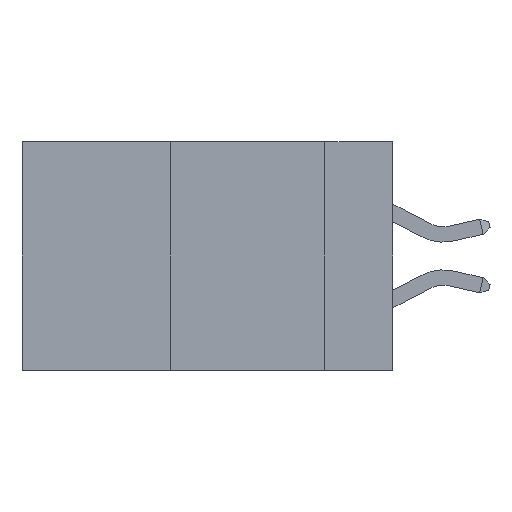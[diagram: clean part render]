
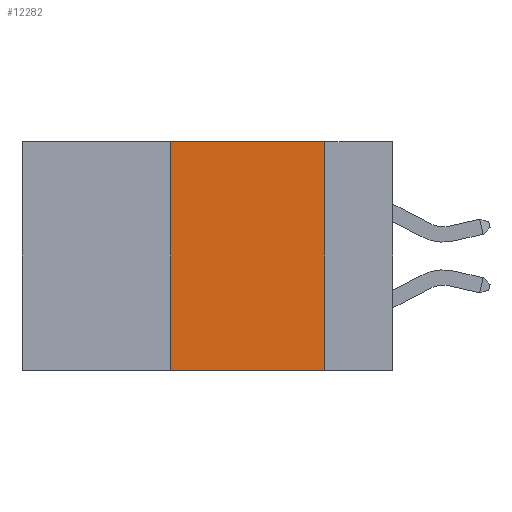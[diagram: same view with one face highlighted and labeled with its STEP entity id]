
A CAD part, left-side view. The second image highlights one B-rep face of the part: STEP entity #12282.
In plain terms, the highlighted planar face has unit normal (-1, 0, 0).
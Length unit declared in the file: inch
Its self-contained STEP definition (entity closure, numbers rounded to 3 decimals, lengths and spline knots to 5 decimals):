
#182 = LINE ( 'NONE', #2516, #6901 ) ;
#681 = CARTESIAN_POINT ( 'NONE',  ( 0., 0.6, -0.37 ) ) ;
#2028 = ORIENTED_EDGE ( 'NONE', *, *, #19809, .F. ) ;
#2516 = CARTESIAN_POINT ( 'NONE',  ( 0., 0.6, 0. ) ) ;
#3698 = VERTEX_POINT ( 'NONE', #8762 ) ;
#4005 = VERTEX_POINT ( 'NONE', #12855 ) ;
#5196 = ORIENTED_EDGE ( 'NONE', *, *, #9722, .F. ) ;
#5280 = ORIENTED_EDGE ( 'NONE', *, *, #16238, .F. ) ;
#5758 = ORIENTED_EDGE ( 'NONE', *, *, #14115, .T. ) ;
#6901 = VECTOR ( 'NONE', #9840, 39.37008 ) ;
#7137 = VERTEX_POINT ( 'NONE', #12231 ) ;
#8507 = PLANE ( 'NONE',  #9341 ) ;
#8762 = CARTESIAN_POINT ( 'NONE',  ( 0., 0.11, -0.37 ) ) ;
#8833 = VECTOR ( 'NONE', #22414, 39.37008 ) ;
#9341 = AXIS2_PLACEMENT_3D ( 'NONE', #16001, #14128, #17877 ) ;
#9382 = LINE ( 'NONE', #16503, #16396 ) ;
#9722 = EDGE_CURVE ( 'NONE', #7137, #4005, #14652, .T. ) ;
#9840 = DIRECTION ( 'NONE',  ( 0., -1., 0. ) ) ;
#11638 = FACE_OUTER_BOUND ( 'NONE', #14631, .T. ) ;
#12231 = CARTESIAN_POINT ( 'NONE',  ( 0., 0.36, -0.37 ) ) ;
#12282 = ADVANCED_FACE ( 'NONE', ( #11638 ), #8507, .F. ) ;
#12676 = DIRECTION ( 'NONE',  ( 0., 0., -1. ) ) ;
#12855 = CARTESIAN_POINT ( 'NONE',  ( 0., 0.36, 0. ) ) ;
#13872 = DIRECTION ( 'NONE',  ( 0., -1., 0. ) ) ;
#14115 = EDGE_CURVE ( 'NONE', #7137, #3698, #17105, .T. ) ;
#14128 = DIRECTION ( 'NONE',  ( 1., 0., 0. ) ) ;
#14631 = EDGE_LOOP ( 'NONE', ( #5280, #2028, #5196, #5758 ) ) ;
#14652 = LINE ( 'NONE', #20379, #8833 ) ;
#15928 = VERTEX_POINT ( 'NONE', #15932 ) ;
#15932 = CARTESIAN_POINT ( 'NONE',  ( 0., 0.11, 0. ) ) ;
#16001 = CARTESIAN_POINT ( 'NONE',  ( 0., 0.6, 0. ) ) ;
#16238 = EDGE_CURVE ( 'NONE', #15928, #3698, #9382, .T. ) ;
#16396 = VECTOR ( 'NONE', #12676, 39.37008 ) ;
#16503 = CARTESIAN_POINT ( 'NONE',  ( 0., 0.11, 0. ) ) ;
#17105 = LINE ( 'NONE', #681, #20299 ) ;
#17877 = DIRECTION ( 'NONE',  ( 0., 0., -1. ) ) ;
#19809 = EDGE_CURVE ( 'NONE', #4005, #15928, #182, .T. ) ;
#20299 = VECTOR ( 'NONE', #13872, 39.37008 ) ;
#20379 = CARTESIAN_POINT ( 'NONE',  ( 0., 0.36, 0. ) ) ;
#22414 = DIRECTION ( 'NONE',  ( 0., 0., 1. ) ) ;
